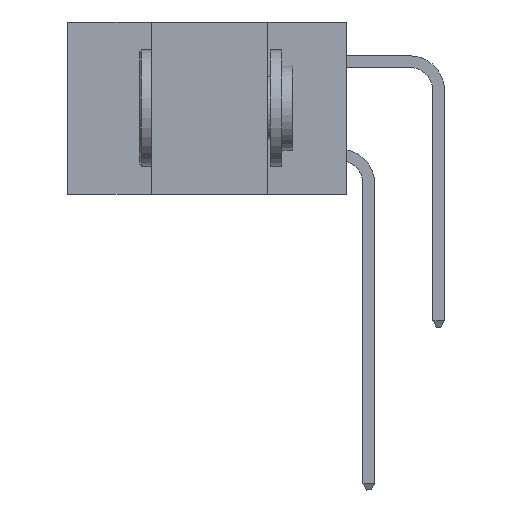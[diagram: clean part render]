
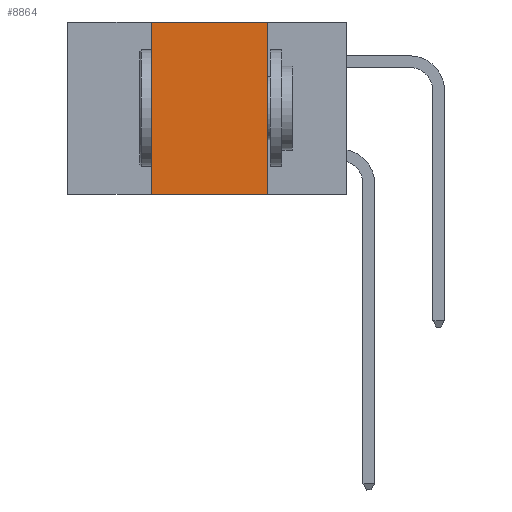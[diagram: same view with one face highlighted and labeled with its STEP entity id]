
A CAD part, left-side view. The second image highlights one B-rep face of the part: STEP entity #8864.
In plain terms, the highlighted planar face has unit normal (-1, 0, 0).
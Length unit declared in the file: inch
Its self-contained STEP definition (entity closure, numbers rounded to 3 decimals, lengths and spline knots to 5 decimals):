
#145 = VERTEX_POINT ( 'NONE', #5786 ) ;
#537 = PLANE ( 'NONE',  #9973 ) ;
#692 = DIRECTION ( 'NONE',  ( 0., 0., 1. ) ) ;
#1569 = DIRECTION ( 'NONE',  ( 0., 0., -1. ) ) ;
#1843 = VECTOR ( 'NONE', #4416, 39.37008 ) ;
#2066 = LINE ( 'NONE', #7400, #11242 ) ;
#2456 = CARTESIAN_POINT ( 'NONE',  ( 0., 0.6, 0. ) ) ;
#2509 = EDGE_CURVE ( 'NONE', #10562, #4414, #8380, .T. ) ;
#3034 = ORIENTED_EDGE ( 'NONE', *, *, #11183, .F. ) ;
#3062 = LINE ( 'NONE', #10829, #8008 ) ;
#3660 = EDGE_CURVE ( 'NONE', #4414, #145, #2066, .T. ) ;
#4030 = ORIENTED_EDGE ( 'NONE', *, *, #3660, .F. ) ;
#4414 = VERTEX_POINT ( 'NONE', #10125 ) ;
#4416 = DIRECTION ( 'NONE',  ( 0., -1., 0. ) ) ;
#5062 = DIRECTION ( 'NONE',  ( 1., 0., 0. ) ) ;
#5786 = CARTESIAN_POINT ( 'NONE',  ( 0., 0.17, 0. ) ) ;
#6040 = CARTESIAN_POINT ( 'NONE',  ( 0., 0.42, 0. ) ) ;
#6529 = ORIENTED_EDGE ( 'NONE', *, *, #2509, .F. ) ;
#6588 = VECTOR ( 'NONE', #692, 39.37008 ) ;
#6915 = ORIENTED_EDGE ( 'NONE', *, *, #7445, .T. ) ;
#7042 = CARTESIAN_POINT ( 'NONE',  ( 0., 0.17, -0.37 ) ) ;
#7143 = CARTESIAN_POINT ( 'NONE',  ( 0., 0.6, -0.37 ) ) ;
#7313 = LINE ( 'NONE', #7143, #1843 ) ;
#7400 = CARTESIAN_POINT ( 'NONE',  ( 0., 0.6, 0. ) ) ;
#7445 = EDGE_CURVE ( 'NONE', #10562, #7958, #7313, .T. ) ;
#7958 = VERTEX_POINT ( 'NONE', #7042 ) ;
#8008 = VECTOR ( 'NONE', #10774, 39.37008 ) ;
#8380 = LINE ( 'NONE', #6040, #6588 ) ;
#8864 = ADVANCED_FACE ( 'NONE', ( #11330 ), #537, .F. ) ;
#8943 = EDGE_LOOP ( 'NONE', ( #3034, #4030, #6529, #6915 ) ) ;
#9973 = AXIS2_PLACEMENT_3D ( 'NONE', #2456, #5062, #1569 ) ;
#10054 = DIRECTION ( 'NONE',  ( 0., -1., 0. ) ) ;
#10125 = CARTESIAN_POINT ( 'NONE',  ( 0., 0.42, 0. ) ) ;
#10129 = CARTESIAN_POINT ( 'NONE',  ( 0., 0.42, -0.37 ) ) ;
#10562 = VERTEX_POINT ( 'NONE', #10129 ) ;
#10774 = DIRECTION ( 'NONE',  ( 0., 0., -1. ) ) ;
#10829 = CARTESIAN_POINT ( 'NONE',  ( 0., 0.17, 0. ) ) ;
#11183 = EDGE_CURVE ( 'NONE', #145, #7958, #3062, .T. ) ;
#11242 = VECTOR ( 'NONE', #10054, 39.37008 ) ;
#11330 = FACE_OUTER_BOUND ( 'NONE', #8943, .T. ) ;
